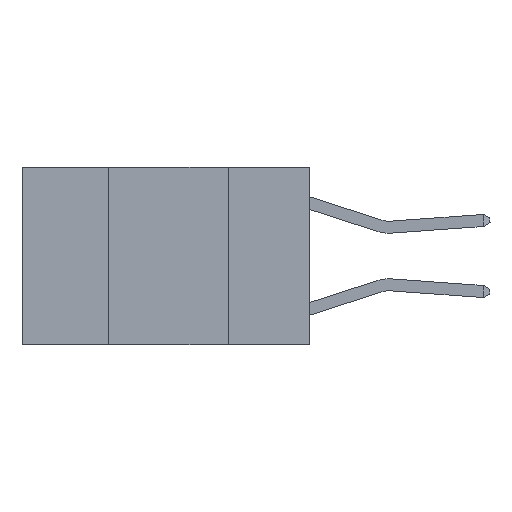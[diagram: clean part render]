
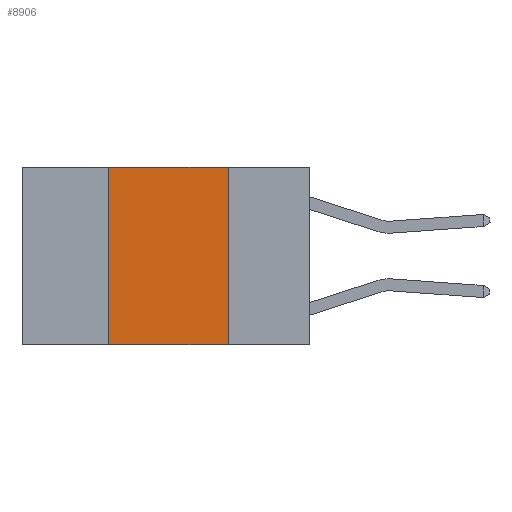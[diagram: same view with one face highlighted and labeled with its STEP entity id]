
A CAD part, left-side view. The second image highlights one B-rep face of the part: STEP entity #8906.
In plain terms, the highlighted planar face has unit normal (-1, 0, 0).
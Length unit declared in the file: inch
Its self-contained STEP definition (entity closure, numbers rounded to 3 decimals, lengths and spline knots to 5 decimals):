
#230 = DIRECTION ( 'NONE',  ( 0., 0., -1. ) ) ;
#1010 = VECTOR ( 'NONE', #1059, 39.37008 ) ;
#1059 = DIRECTION ( 'NONE',  ( 0., 0., 1. ) ) ;
#1554 = EDGE_LOOP ( 'NONE', ( #7393, #10963, #14049, #8519 ) ) ;
#2835 = FACE_OUTER_BOUND ( 'NONE', #1554, .T. ) ;
#3285 = CARTESIAN_POINT ( 'NONE',  ( 0., 0.17, -0.37 ) ) ;
#3615 = EDGE_CURVE ( 'NONE', #12494, #9296, #12171, .T. ) ;
#3782 = PLANE ( 'NONE',  #5709 ) ;
#4144 = CARTESIAN_POINT ( 'NONE',  ( 0., 0.17, 0. ) ) ;
#4308 = EDGE_CURVE ( 'NONE', #12494, #13768, #6413, .T. ) ;
#4533 = CARTESIAN_POINT ( 'NONE',  ( 0., 0.6, 0. ) ) ;
#5028 = DIRECTION ( 'NONE',  ( 1., 0., 0. ) ) ;
#5303 = CARTESIAN_POINT ( 'NONE',  ( 0., 0.17, 0. ) ) ;
#5596 = DIRECTION ( 'NONE',  ( 0., -1., 0. ) ) ;
#5709 = AXIS2_PLACEMENT_3D ( 'NONE', #14429, #5028, #13291 ) ;
#5791 = CARTESIAN_POINT ( 'NONE',  ( 0., 0.6, -0.37 ) ) ;
#5974 = CARTESIAN_POINT ( 'NONE',  ( 0., 0.42, -0.37 ) ) ;
#6413 = LINE ( 'NONE', #7159, #1010 ) ;
#6937 = LINE ( 'NONE', #4533, #9816 ) ;
#7159 = CARTESIAN_POINT ( 'NONE',  ( 0., 0.42, 0. ) ) ;
#7393 = ORIENTED_EDGE ( 'NONE', *, *, #14135, .F. ) ;
#7521 = VECTOR ( 'NONE', #230, 39.37008 ) ;
#7897 = LINE ( 'NONE', #5303, #7521 ) ;
#8519 = ORIENTED_EDGE ( 'NONE', *, *, #3615, .T. ) ;
#8659 = VECTOR ( 'NONE', #5596, 39.37008 ) ;
#8906 = ADVANCED_FACE ( 'NONE', ( #2835 ), #3782, .F. ) ;
#9296 = VERTEX_POINT ( 'NONE', #3285 ) ;
#9403 = CARTESIAN_POINT ( 'NONE',  ( 0., 0.42, 0. ) ) ;
#9614 = VERTEX_POINT ( 'NONE', #4144 ) ;
#9816 = VECTOR ( 'NONE', #13994, 39.37008 ) ;
#10963 = ORIENTED_EDGE ( 'NONE', *, *, #14345, .F. ) ;
#12171 = LINE ( 'NONE', #5791, #8659 ) ;
#12494 = VERTEX_POINT ( 'NONE', #5974 ) ;
#13291 = DIRECTION ( 'NONE',  ( 0., 0., -1. ) ) ;
#13768 = VERTEX_POINT ( 'NONE', #9403 ) ;
#13994 = DIRECTION ( 'NONE',  ( 0., -1., 0. ) ) ;
#14049 = ORIENTED_EDGE ( 'NONE', *, *, #4308, .F. ) ;
#14135 = EDGE_CURVE ( 'NONE', #9614, #9296, #7897, .T. ) ;
#14345 = EDGE_CURVE ( 'NONE', #13768, #9614, #6937, .T. ) ;
#14429 = CARTESIAN_POINT ( 'NONE',  ( 0., 0.6, 0. ) ) ;
